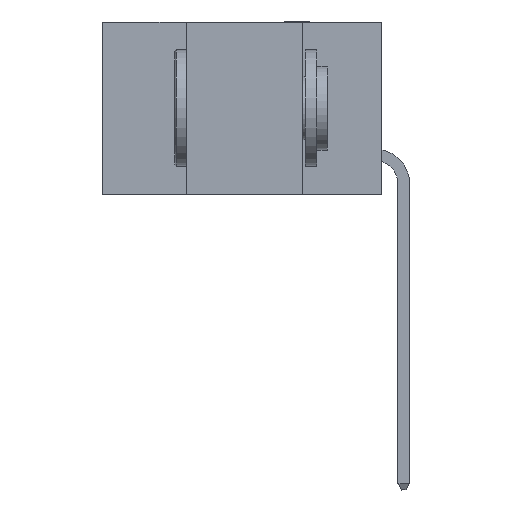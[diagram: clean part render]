
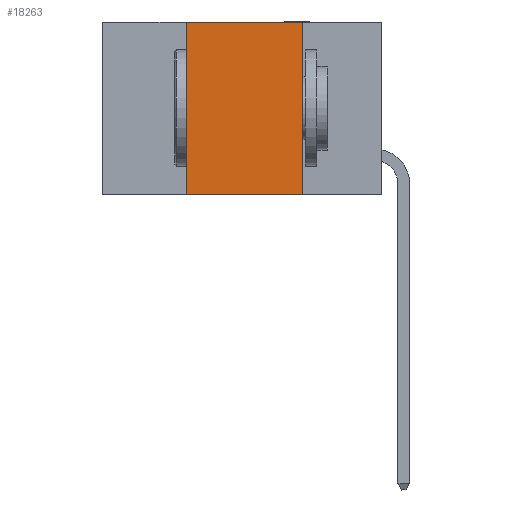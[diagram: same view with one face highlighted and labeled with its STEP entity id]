
A CAD part, left-side view. The second image highlights one B-rep face of the part: STEP entity #18263.
In plain terms, the highlighted planar face has unit normal (-1, 0, 0).
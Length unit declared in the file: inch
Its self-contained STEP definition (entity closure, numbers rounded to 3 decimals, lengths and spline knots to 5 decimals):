
#14 = CARTESIAN_POINT ( 'NONE',  ( 0., 0.42, 0. ) ) ;
#719 = DIRECTION ( 'NONE',  ( 0., 0., -1. ) ) ;
#771 = CARTESIAN_POINT ( 'NONE',  ( 0., 0.42, -0.37 ) ) ;
#919 = VERTEX_POINT ( 'NONE', #18677 ) ;
#1843 = FACE_OUTER_BOUND ( 'NONE', #7590, .T. ) ;
#2037 = VECTOR ( 'NONE', #33176, 39.37008 ) ;
#3606 = DIRECTION ( 'NONE',  ( 0., 0., 1. ) ) ;
#6115 = CARTESIAN_POINT ( 'NONE',  ( 0., 0.17, 0. ) ) ;
#6300 = VECTOR ( 'NONE', #719, 39.37008 ) ;
#7336 = ORIENTED_EDGE ( 'NONE', *, *, #28120, .T. ) ;
#7569 = EDGE_CURVE ( 'NONE', #23745, #8134, #8927, .T. ) ;
#7590 = EDGE_LOOP ( 'NONE', ( #29800, #19627, #7994, #7336 ) ) ;
#7700 = DIRECTION ( 'NONE',  ( 0., -1., 0. ) ) ;
#7994 = ORIENTED_EDGE ( 'NONE', *, *, #7569, .F. ) ;
#8124 = LINE ( 'NONE', #15184, #2037 ) ;
#8134 = VERTEX_POINT ( 'NONE', #14 ) ;
#8927 = LINE ( 'NONE', #19234, #9767 ) ;
#9085 = DIRECTION ( 'NONE',  ( 1., 0., 0. ) ) ;
#9767 = VECTOR ( 'NONE', #3606, 39.37008 ) ;
#10249 = EDGE_CURVE ( 'NONE', #32738, #919, #13256, .T. ) ;
#10688 = VECTOR ( 'NONE', #7700, 39.37008 ) ;
#11537 = EDGE_CURVE ( 'NONE', #8134, #32738, #29774, .T. ) ;
#13256 = LINE ( 'NONE', #29485, #6300 ) ;
#15184 = CARTESIAN_POINT ( 'NONE',  ( 0., 0.6, -0.37 ) ) ;
#15661 = AXIS2_PLACEMENT_3D ( 'NONE', #19469, #9085, #29880 ) ;
#18263 = ADVANCED_FACE ( 'NONE', ( #1843 ), #29777, .F. ) ;
#18677 = CARTESIAN_POINT ( 'NONE',  ( 0., 0.17, -0.37 ) ) ;
#19234 = CARTESIAN_POINT ( 'NONE',  ( 0., 0.42, 0. ) ) ;
#19469 = CARTESIAN_POINT ( 'NONE',  ( 0., 0.6, 0. ) ) ;
#19627 = ORIENTED_EDGE ( 'NONE', *, *, #11537, .F. ) ;
#23745 = VERTEX_POINT ( 'NONE', #771 ) ;
#28120 = EDGE_CURVE ( 'NONE', #23745, #919, #8124, .T. ) ;
#29485 = CARTESIAN_POINT ( 'NONE',  ( 0., 0.17, 0. ) ) ;
#29774 = LINE ( 'NONE', #33388, #10688 ) ;
#29777 = PLANE ( 'NONE',  #15661 ) ;
#29800 = ORIENTED_EDGE ( 'NONE', *, *, #10249, .F. ) ;
#29880 = DIRECTION ( 'NONE',  ( 0., 0., -1. ) ) ;
#32738 = VERTEX_POINT ( 'NONE', #6115 ) ;
#33176 = DIRECTION ( 'NONE',  ( 0., -1., 0. ) ) ;
#33388 = CARTESIAN_POINT ( 'NONE',  ( 0., 0.6, 0. ) ) ;
